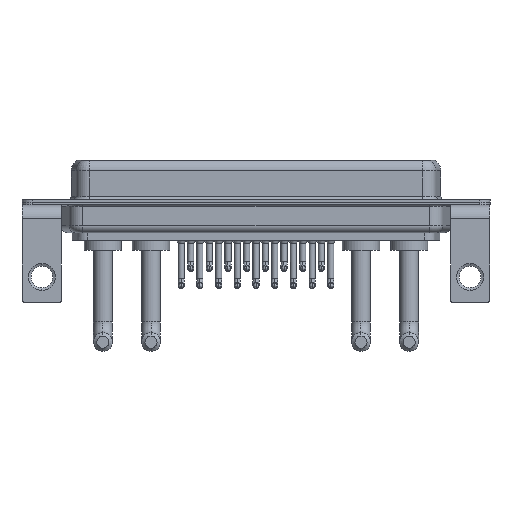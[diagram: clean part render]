
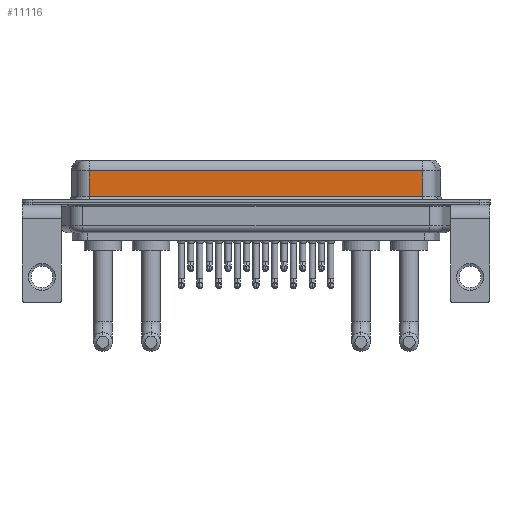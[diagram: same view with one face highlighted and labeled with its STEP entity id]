
A CAD part, front view. The second image highlights one B-rep face of the part: STEP entity #11116.
In plain terms, the highlighted planar face has unit normal (0, -1, 0).
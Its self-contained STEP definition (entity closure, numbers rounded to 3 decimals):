
#688 = VERTEX_POINT ( 'NONE', #7160 ) ;
#779 = VERTEX_POINT ( 'NONE', #12681 ) ;
#1207 = VERTEX_POINT ( 'NONE', #21077 ) ;
#1241 = DIRECTION ( 'NONE',  ( 0., 0., -1. ) ) ;
#1392 = VERTEX_POINT ( 'NONE', #10175 ) ;
#1497 = CARTESIAN_POINT ( 'NONE',  ( 7.038, -3.95, 6.4 ) ) ;
#3631 = EDGE_CURVE ( 'NONE', #1207, #779, #19550, .T. ) ;
#3728 = DIRECTION ( 'NONE',  ( -1., 0., 0. ) ) ;
#5041 = FACE_OUTER_BOUND ( 'NONE', #15516, .T. ) ;
#5273 = LINE ( 'NONE', #19367, #12106 ) ;
#5290 = PLANE ( 'NONE',  #11857 ) ;
#5562 = ORIENTED_EDGE ( 'NONE', *, *, #18933, .F. ) ;
#7160 = CARTESIAN_POINT ( 'NONE',  ( 56.462, -3.95, 0.9 ) ) ;
#7230 = DIRECTION ( 'NONE',  ( 1., 0., 0. ) ) ;
#8627 = EDGE_CURVE ( 'NONE', #779, #1392, #15226, .T. ) ;
#9765 = CARTESIAN_POINT ( 'NONE',  ( 56.462, -3.95, 6.4 ) ) ;
#10175 = CARTESIAN_POINT ( 'NONE',  ( 7.038, -3.95, 0.9 ) ) ;
#10696 = DIRECTION ( 'NONE',  ( 0., 1., 0. ) ) ;
#11116 = ADVANCED_FACE ( 'NONE', ( #5041 ), #5290, .F. ) ;
#11857 = AXIS2_PLACEMENT_3D ( 'NONE', #17774, #10696, #19498 ) ;
#12106 = VECTOR ( 'NONE', #7230, 1000. ) ;
#12681 = CARTESIAN_POINT ( 'NONE',  ( 7.038, -3.95, 4.65 ) ) ;
#13640 = ORIENTED_EDGE ( 'NONE', *, *, #19074, .T. ) ;
#14329 = VECTOR ( 'NONE', #1241, 1000. ) ;
#14330 = CARTESIAN_POINT ( 'NONE',  ( 56.462, -3.95, 4.65 ) ) ;
#14722 = VECTOR ( 'NONE', #22263, 1000. ) ;
#15226 = LINE ( 'NONE', #1497, #14722 ) ;
#15516 = EDGE_LOOP ( 'NONE', ( #5562, #18001, #20411, #13640 ) ) ;
#16164 = VECTOR ( 'NONE', #3728, 1000. ) ;
#17063 = LINE ( 'NONE', #9765, #14329 ) ;
#17774 = CARTESIAN_POINT ( 'NONE',  ( 56.462, -3.95, 6.4 ) ) ;
#18001 = ORIENTED_EDGE ( 'NONE', *, *, #3631, .T. ) ;
#18933 = EDGE_CURVE ( 'NONE', #1207, #688, #17063, .T. ) ;
#19074 = EDGE_CURVE ( 'NONE', #1392, #688, #5273, .T. ) ;
#19367 = CARTESIAN_POINT ( 'NONE',  ( 56.462, -3.95, 0.9 ) ) ;
#19498 = DIRECTION ( 'NONE',  ( 0., 0., 1. ) ) ;
#19550 = LINE ( 'NONE', #14330, #16164 ) ;
#20411 = ORIENTED_EDGE ( 'NONE', *, *, #8627, .T. ) ;
#21077 = CARTESIAN_POINT ( 'NONE',  ( 56.462, -3.95, 4.65 ) ) ;
#22263 = DIRECTION ( 'NONE',  ( 0., 0., -1. ) ) ;
